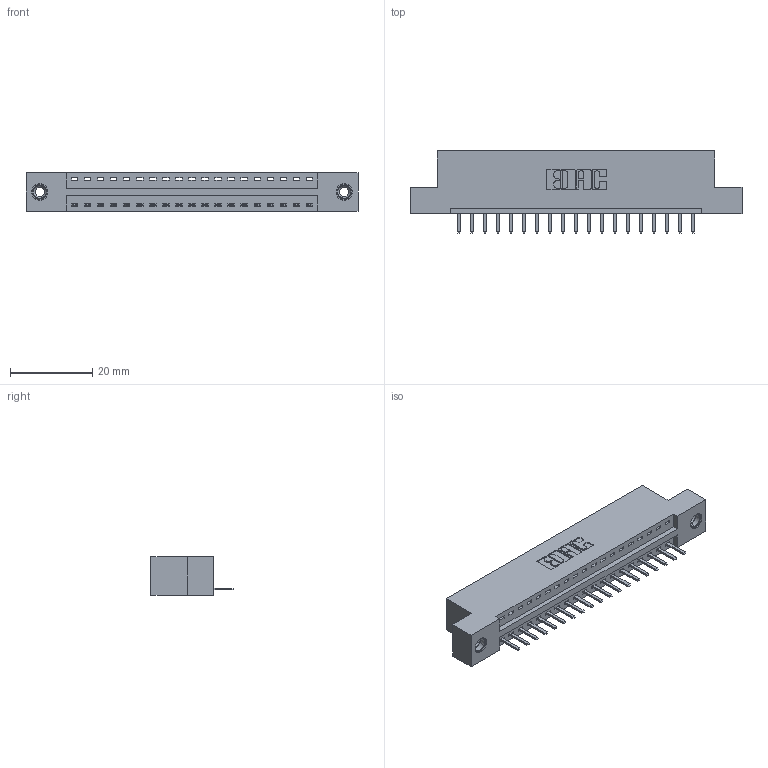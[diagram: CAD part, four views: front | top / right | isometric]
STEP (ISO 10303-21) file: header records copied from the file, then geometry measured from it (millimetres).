
FILE_DESCRIPTION (( 'STEP AP203' ), '1' );
FILE_NAME ('396-019-520-108.STEP', '2019-10-26T20:13:28', ( '' ), ( '' ), 'SwSTEP 2.0', 'SolidWorks 2016', '' );
FILE_SCHEMA (( 'CONFIG_CONTROL_DESIGN' ));
Length unit declared in the file: inch
Products named in the file (4): 345-292-001_345-293-120; 396-019-520-108; 346 Part_Flush Mounting Lugs - 0.156 Dia-TI; 345-250-001_345-250-003-102
Assembly tree (22 placements, depth 2):
  396-019-520-108
    346 Part_Flush Mounting Lugs - 0.156 Dia-TI
    345-292-001_345-293-120  x19
    345-250-001_345-250-003-102  x2
Bounding box: 80.9 x 20.02 x 9.4 mm (x, y, z)
Volume: 7524.2 mm3; surface area: 8995.4 mm2
Topology: 22 solids, 22 shells, 1360 faces, 3961 edges, 2582 vertices
Faces by surface type: plane 906, cylinder 438, cone 12, torus 4
Entity records: 16188 total; most frequent: CARTESIAN_POINT 2776, ORIENTED_EDGE 2710, DIRECTION 2491, EDGE_CURVE 1355, VECTOR 1123, LINE 1123, VERTEX_POINT 896, AXIS2_PLACEMENT_3D 684
